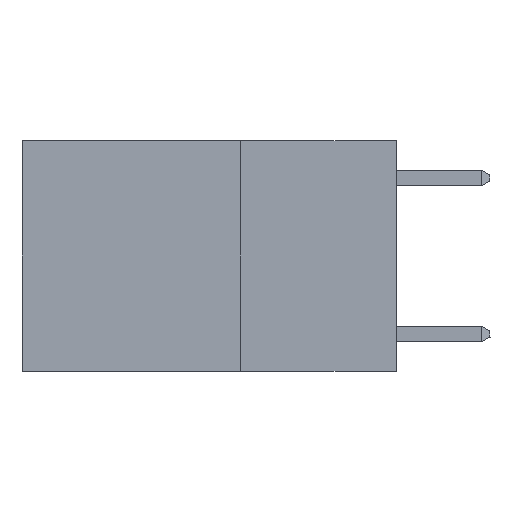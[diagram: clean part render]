
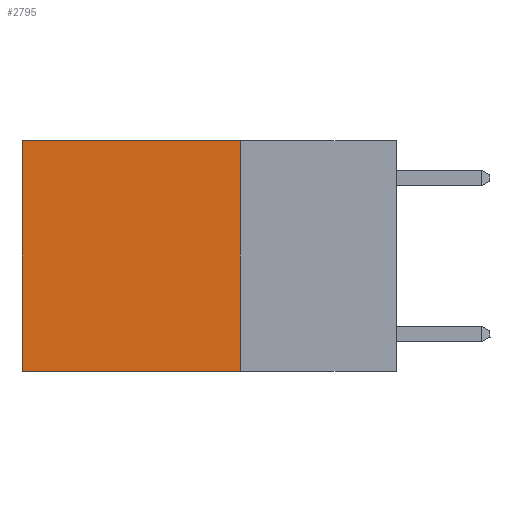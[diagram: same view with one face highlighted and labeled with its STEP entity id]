
A CAD part, left-side view. The second image highlights one B-rep face of the part: STEP entity #2795.
In plain terms, the highlighted planar face has unit normal (-1, 0, 0).
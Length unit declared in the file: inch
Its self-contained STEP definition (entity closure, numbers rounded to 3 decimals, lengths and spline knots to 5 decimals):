
#14 = LINE ( 'NONE', #4208, #6085 ) ;
#136 = CARTESIAN_POINT ( 'NONE',  ( 0.2625, 0.25, -0.37 ) ) ;
#175 = VERTEX_POINT ( 'NONE', #5507 ) ;
#239 = EDGE_CURVE ( 'NONE', #14093, #175, #14, .T. ) ;
#423 = VECTOR ( 'NONE', #8535, 39.37008 ) ;
#1300 = EDGE_CURVE ( 'NONE', #3785, #2618, #13371, .T. ) ;
#2433 = LINE ( 'NONE', #5460, #11500 ) ;
#2618 = VERTEX_POINT ( 'NONE', #6704 ) ;
#2795 = ADVANCED_FACE ( 'NONE', ( #8215 ), #4753, .F. ) ;
#3785 = VERTEX_POINT ( 'NONE', #10190 ) ;
#4208 = CARTESIAN_POINT ( 'NONE',  ( 0.2625, 0.6, 0. ) ) ;
#4474 = VECTOR ( 'NONE', #8262, 39.37008 ) ;
#4753 = PLANE ( 'NONE',  #11679 ) ;
#5460 = CARTESIAN_POINT ( 'NONE',  ( 0.2625, 0.25, 0. ) ) ;
#5507 = CARTESIAN_POINT ( 'NONE',  ( 0.2625, 0.6, -0.37 ) ) ;
#6079 = EDGE_LOOP ( 'NONE', ( #11422, #11752, #12318, #12328 ) ) ;
#6085 = VECTOR ( 'NONE', #13770, 39.37008 ) ;
#6115 = DIRECTION ( 'NONE',  ( 1., 0., 0. ) ) ;
#6704 = CARTESIAN_POINT ( 'NONE',  ( 0.2625, 0.25, -0.37 ) ) ;
#6720 = DIRECTION ( 'NONE',  ( 0., 1., 0. ) ) ;
#7700 = CARTESIAN_POINT ( 'NONE',  ( 0.2625, 0.25, 0. ) ) ;
#8215 = FACE_OUTER_BOUND ( 'NONE', #6079, .T. ) ;
#8262 = DIRECTION ( 'NONE',  ( 0., 0., -1. ) ) ;
#8535 = DIRECTION ( 'NONE',  ( 0., 1., 0. ) ) ;
#8978 = EDGE_CURVE ( 'NONE', #3785, #14093, #2433, .T. ) ;
#10190 = CARTESIAN_POINT ( 'NONE',  ( 0.2625, 0.25, 0. ) ) ;
#10721 = CARTESIAN_POINT ( 'NONE',  ( 0.2625, 0.25, 0. ) ) ;
#11422 = ORIENTED_EDGE ( 'NONE', *, *, #239, .T. ) ;
#11500 = VECTOR ( 'NONE', #6720, 39.37008 ) ;
#11679 = AXIS2_PLACEMENT_3D ( 'NONE', #10721, #6115, #14040 ) ;
#11752 = ORIENTED_EDGE ( 'NONE', *, *, #13925, .F. ) ;
#12318 = ORIENTED_EDGE ( 'NONE', *, *, #1300, .F. ) ;
#12328 = ORIENTED_EDGE ( 'NONE', *, *, #8978, .T. ) ;
#12920 = LINE ( 'NONE', #136, #423 ) ;
#13153 = CARTESIAN_POINT ( 'NONE',  ( 0.2625, 0.6, 0. ) ) ;
#13371 = LINE ( 'NONE', #7700, #4474 ) ;
#13770 = DIRECTION ( 'NONE',  ( 0., 0., -1. ) ) ;
#13925 = EDGE_CURVE ( 'NONE', #2618, #175, #12920, .T. ) ;
#14040 = DIRECTION ( 'NONE',  ( 0., 0., -1. ) ) ;
#14093 = VERTEX_POINT ( 'NONE', #13153 ) ;
